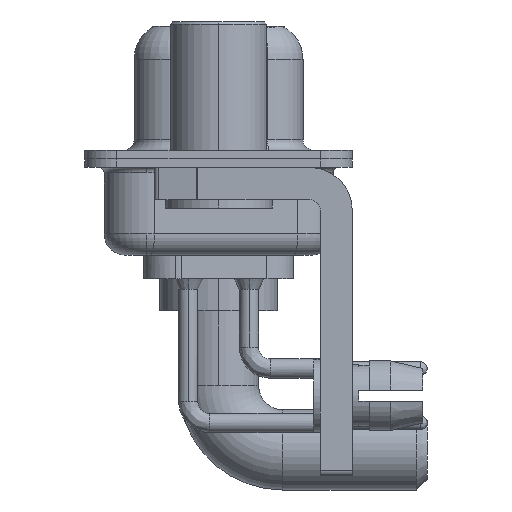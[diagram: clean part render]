
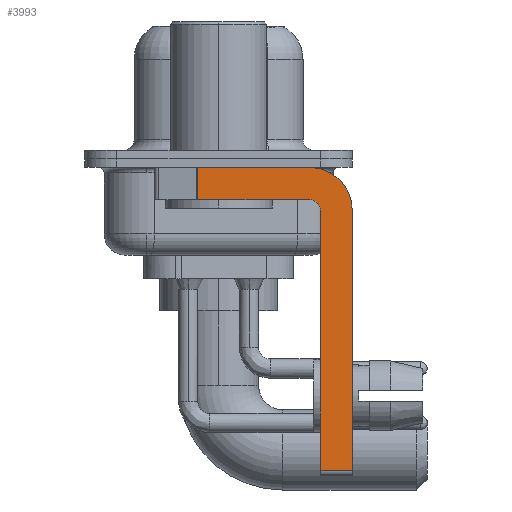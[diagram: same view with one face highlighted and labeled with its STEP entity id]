
A CAD part, left-side view. The second image highlights one B-rep face of the part: STEP entity #3993.
In plain terms, the highlighted planar face has unit normal (-1, 0, 0).
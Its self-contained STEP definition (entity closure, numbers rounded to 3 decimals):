
#334 = CARTESIAN_POINT ( 'NONE',  ( -2.9, -4.25, -2.4 ) ) ;
#693 = DIRECTION ( 'NONE',  ( 0., 0., -1. ) ) ;
#775 = EDGE_CURVE ( 'NONE', #4472, #2831, #20714, .T. ) ;
#936 = DIRECTION ( 'NONE',  ( -1., 0., 0. ) ) ;
#1117 = CARTESIAN_POINT ( 'NONE',  ( -2.9, 0.978, -1.9 ) ) ;
#1343 = ORIENTED_EDGE ( 'NONE', *, *, #18838, .T. ) ;
#1415 = CARTESIAN_POINT ( 'NONE',  ( -2.9, -4.25, -0.4 ) ) ;
#1819 = VERTEX_POINT ( 'NONE', #21083 ) ;
#1976 = CARTESIAN_POINT ( 'NONE',  ( -2.9, -4.25, -2.4 ) ) ;
#2400 = CARTESIAN_POINT ( 'NONE',  ( -2.9, 3., -0.4 ) ) ;
#2705 = VECTOR ( 'NONE', #693, 1000. ) ;
#2831 = VERTEX_POINT ( 'NONE', #16553 ) ;
#2934 = EDGE_CURVE ( 'NONE', #1819, #4472, #14898, .T. ) ;
#2944 = EDGE_LOOP ( 'NONE', ( #9439, #13723, #21496, #5387, #18881, #1343, #14636, #20479 ) ) ;
#3338 = DIRECTION ( 'NONE',  ( 1., 0., 0. ) ) ;
#3540 = DIRECTION ( 'NONE',  ( 1., 0., 0. ) ) ;
#3993 = ADVANCED_FACE ( 'NONE', ( #17082 ), #8655, .F. ) ;
#4472 = VERTEX_POINT ( 'NONE', #12089 ) ;
#5246 = CARTESIAN_POINT ( 'NONE',  ( -2.9, 0.978, -0.4 ) ) ;
#5387 = ORIENTED_EDGE ( 'NONE', *, *, #775, .F. ) ;
#5789 = VECTOR ( 'NONE', #10834, 1000. ) ;
#6252 = VERTEX_POINT ( 'NONE', #5246 ) ;
#6372 = VERTEX_POINT ( 'NONE', #19217 ) ;
#6509 = VECTOR ( 'NONE', #15001, 1000. ) ;
#8239 = EDGE_CURVE ( 'NONE', #12465, #6372, #10532, .T. ) ;
#8655 = PLANE ( 'NONE',  #16091 ) ;
#9439 = ORIENTED_EDGE ( 'NONE', *, *, #16289, .F. ) ;
#9814 = CARTESIAN_POINT ( 'NONE',  ( -2.9, -4.25, -2.4 ) ) ;
#9883 = DIRECTION ( 'NONE',  ( 0., 0., -1. ) ) ;
#10328 = DIRECTION ( 'NONE',  ( 0., 0., -1. ) ) ;
#10337 = VECTOR ( 'NONE', #9883, 1000. ) ;
#10532 = CIRCLE ( 'NONE', #21214, 2. ) ;
#10790 = LINE ( 'NONE', #17333, #2705 ) ;
#10834 = DIRECTION ( 'NONE',  ( 0., -1., 0. ) ) ;
#11108 = LINE ( 'NONE', #1117, #10337 ) ;
#12089 = CARTESIAN_POINT ( 'NONE',  ( -2.9, -4.75, -2.4 ) ) ;
#12465 = VERTEX_POINT ( 'NONE', #1415 ) ;
#12982 = VECTOR ( 'NONE', #20295, 1000. ) ;
#13553 = CARTESIAN_POINT ( 'NONE',  ( -2.9, -4.25, -1.9 ) ) ;
#13723 = ORIENTED_EDGE ( 'NONE', *, *, #15165, .T. ) ;
#13810 = CARTESIAN_POINT ( 'NONE',  ( -2.9, -4.25, -14.55 ) ) ;
#13936 = AXIS2_PLACEMENT_3D ( 'NONE', #9814, #936, #16576 ) ;
#14636 = ORIENTED_EDGE ( 'NONE', *, *, #19423, .F. ) ;
#14898 = LINE ( 'NONE', #21694, #6509 ) ;
#15001 = DIRECTION ( 'NONE',  ( 0., 0., 1. ) ) ;
#15122 = VECTOR ( 'NONE', #20138, 1000. ) ;
#15165 = EDGE_CURVE ( 'NONE', #6252, #16840, #11108, .T. ) ;
#16091 = AXIS2_PLACEMENT_3D ( 'NONE', #334, #3338, #10328 ) ;
#16104 = CARTESIAN_POINT ( 'NONE',  ( -2.9, 0.978, -1.9 ) ) ;
#16289 = EDGE_CURVE ( 'NONE', #6252, #12465, #20970, .T. ) ;
#16553 = CARTESIAN_POINT ( 'NONE',  ( -2.9, -4.25, -1.9 ) ) ;
#16576 = DIRECTION ( 'NONE',  ( 0., 0., 1. ) ) ;
#16840 = VERTEX_POINT ( 'NONE', #16104 ) ;
#17082 = FACE_OUTER_BOUND ( 'NONE', #2944, .T. ) ;
#17241 = CARTESIAN_POINT ( 'NONE',  ( -2.9, -6.25, -14.55 ) ) ;
#17333 = CARTESIAN_POINT ( 'NONE',  ( -2.9, -6.25, -2.4 ) ) ;
#18608 = LINE ( 'NONE', #13810, #12982 ) ;
#18838 = EDGE_CURVE ( 'NONE', #1819, #21899, #18608, .T. ) ;
#18881 = ORIENTED_EDGE ( 'NONE', *, *, #2934, .F. ) ;
#19217 = CARTESIAN_POINT ( 'NONE',  ( -2.9, -6.25, -2.4 ) ) ;
#19423 = EDGE_CURVE ( 'NONE', #6372, #21899, #10790, .T. ) ;
#20138 = DIRECTION ( 'NONE',  ( 0., 1., 0. ) ) ;
#20295 = DIRECTION ( 'NONE',  ( 0., -1., 0. ) ) ;
#20479 = ORIENTED_EDGE ( 'NONE', *, *, #8239, .F. ) ;
#20554 = DIRECTION ( 'NONE',  ( 0., 0., -1. ) ) ;
#20714 = CIRCLE ( 'NONE', #13936, 0.5 ) ;
#20970 = LINE ( 'NONE', #2400, #5789 ) ;
#21083 = CARTESIAN_POINT ( 'NONE',  ( -2.9, -4.75, -14.55 ) ) ;
#21120 = EDGE_CURVE ( 'NONE', #2831, #16840, #21920, .T. ) ;
#21214 = AXIS2_PLACEMENT_3D ( 'NONE', #1976, #3540, #20554 ) ;
#21496 = ORIENTED_EDGE ( 'NONE', *, *, #21120, .F. ) ;
#21694 = CARTESIAN_POINT ( 'NONE',  ( -2.9, -4.75, -14.8 ) ) ;
#21899 = VERTEX_POINT ( 'NONE', #17241 ) ;
#21920 = LINE ( 'NONE', #13553, #15122 ) ;
